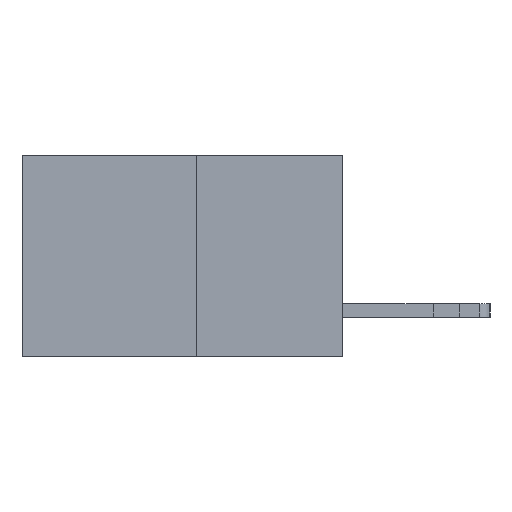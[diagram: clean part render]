
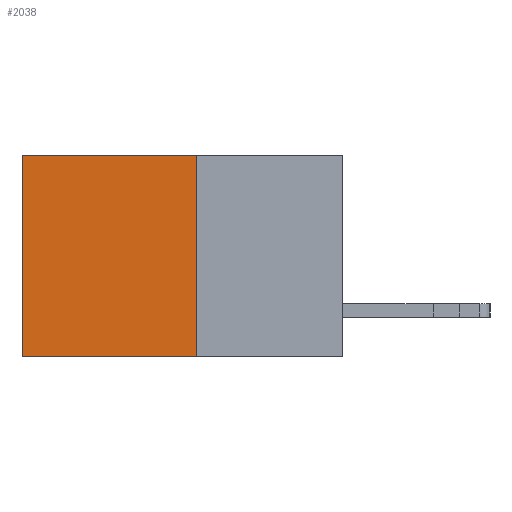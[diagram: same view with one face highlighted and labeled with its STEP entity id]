
A CAD part, left-side view. The second image highlights one B-rep face of the part: STEP entity #2038.
In plain terms, the highlighted planar face has unit normal (-1, 0, 0).
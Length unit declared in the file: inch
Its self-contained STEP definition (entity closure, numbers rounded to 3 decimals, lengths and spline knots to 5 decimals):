
#68 = CARTESIAN_POINT ( 'NONE',  ( 0.277, 0.27, 0. ) ) ;
#936 = EDGE_CURVE ( 'NONE', #6184, #8985, #4330, .T. ) ;
#1117 = ORIENTED_EDGE ( 'NONE', *, *, #1158, .T. ) ;
#1158 = EDGE_CURVE ( 'NONE', #8985, #4743, #1513, .T. ) ;
#1420 = DIRECTION ( 'NONE',  ( 0., 0., -1. ) ) ;
#1513 = LINE ( 'NONE', #2053, #11548 ) ;
#2038 = ADVANCED_FACE ( 'NONE', ( #8978 ), #3439, .F. ) ;
#2053 = CARTESIAN_POINT ( 'NONE',  ( 0.277, 0.59, -0.37 ) ) ;
#2518 = LINE ( 'NONE', #11792, #11929 ) ;
#3003 = ORIENTED_EDGE ( 'NONE', *, *, #936, .T. ) ;
#3439 = PLANE ( 'NONE',  #10799 ) ;
#3816 = LINE ( 'NONE', #11038, #11224 ) ;
#4066 = EDGE_CURVE ( 'NONE', #5164, #4743, #2518, .T. ) ;
#4330 = LINE ( 'NONE', #5973, #6922 ) ;
#4561 = CARTESIAN_POINT ( 'NONE',  ( 0.277, 0.27, -0.37 ) ) ;
#4743 = VERTEX_POINT ( 'NONE', #9722 ) ;
#4872 = CARTESIAN_POINT ( 'NONE',  ( 0.277, 0.27, -0.37 ) ) ;
#5164 = VERTEX_POINT ( 'NONE', #4872 ) ;
#5973 = CARTESIAN_POINT ( 'NONE',  ( 0.277, 0.27, 0. ) ) ;
#6019 = EDGE_CURVE ( 'NONE', #6184, #5164, #3816, .T. ) ;
#6184 = VERTEX_POINT ( 'NONE', #68 ) ;
#6196 = ORIENTED_EDGE ( 'NONE', *, *, #6019, .F. ) ;
#6352 = ORIENTED_EDGE ( 'NONE', *, *, #4066, .F. ) ;
#6428 = DIRECTION ( 'NONE',  ( 1., 0., 0. ) ) ;
#6922 = VECTOR ( 'NONE', #9272, 39.37008 ) ;
#8978 = FACE_OUTER_BOUND ( 'NONE', #11337, .T. ) ;
#8985 = VERTEX_POINT ( 'NONE', #9130 ) ;
#9130 = CARTESIAN_POINT ( 'NONE',  ( 0.277, 0.59, 0. ) ) ;
#9272 = DIRECTION ( 'NONE',  ( 0., 1., 0. ) ) ;
#9722 = CARTESIAN_POINT ( 'NONE',  ( 0.277, 0.59, -0.37 ) ) ;
#9914 = DIRECTION ( 'NONE',  ( 0., 0., -1. ) ) ;
#10799 = AXIS2_PLACEMENT_3D ( 'NONE', #4561, #6428, #1420 ) ;
#11038 = CARTESIAN_POINT ( 'NONE',  ( 0.277, 0.27, -0.37 ) ) ;
#11062 = DIRECTION ( 'NONE',  ( 0., 0., -1. ) ) ;
#11224 = VECTOR ( 'NONE', #11062, 39.37008 ) ;
#11337 = EDGE_LOOP ( 'NONE', ( #1117, #6352, #6196, #3003 ) ) ;
#11548 = VECTOR ( 'NONE', #9914, 39.37008 ) ;
#11792 = CARTESIAN_POINT ( 'NONE',  ( 0.277, 0.27, -0.37 ) ) ;
#11929 = VECTOR ( 'NONE', #12118, 39.37008 ) ;
#12118 = DIRECTION ( 'NONE',  ( 0., 1., 0. ) ) ;
